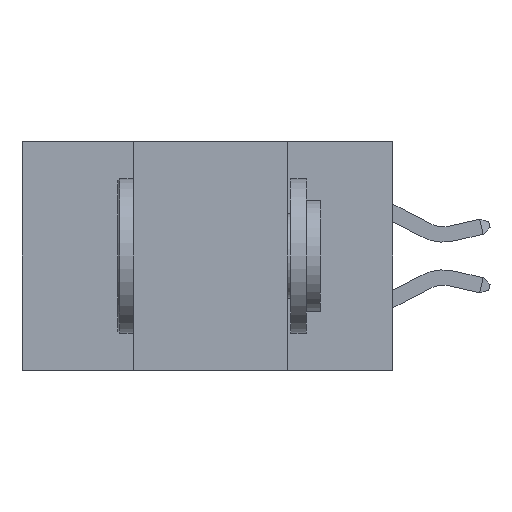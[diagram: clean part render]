
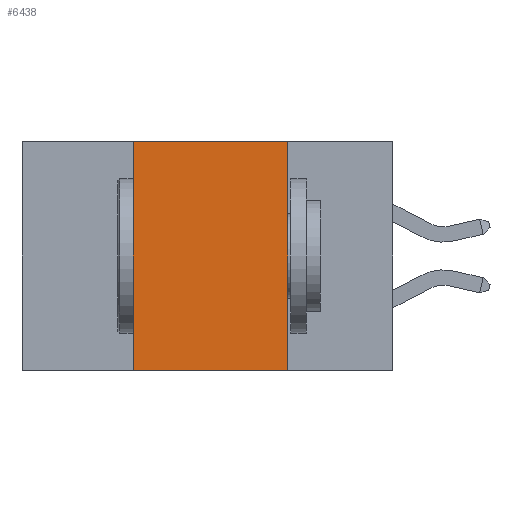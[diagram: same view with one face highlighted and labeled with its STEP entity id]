
A CAD part, left-side view. The second image highlights one B-rep face of the part: STEP entity #6438.
In plain terms, the highlighted planar face has unit normal (-1, 0, 0).
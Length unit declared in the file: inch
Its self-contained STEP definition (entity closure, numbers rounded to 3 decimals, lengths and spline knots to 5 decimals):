
#1858 = VERTEX_POINT ( 'NONE', #30913 ) ;
#2085 = DIRECTION ( 'NONE',  ( 0., 0., -1. ) ) ;
#2161 = VECTOR ( 'NONE', #22257, 39.37008 ) ;
#2575 = CARTESIAN_POINT ( 'NONE',  ( 0., 0.17, 0. ) ) ;
#4221 = DIRECTION ( 'NONE',  ( 0., 0., 1. ) ) ;
#5257 = DIRECTION ( 'NONE',  ( 0., 0., -1. ) ) ;
#6438 = ADVANCED_FACE ( 'NONE', ( #17389 ), #26666, .F. ) ;
#7757 = DIRECTION ( 'NONE',  ( 0., -1., 0. ) ) ;
#9501 = VECTOR ( 'NONE', #7757, 39.37008 ) ;
#10802 = VERTEX_POINT ( 'NONE', #17615 ) ;
#10861 = EDGE_CURVE ( 'NONE', #1858, #30908, #12055, .T. ) ;
#11122 = ORIENTED_EDGE ( 'NONE', *, *, #29031, .T. ) ;
#12055 = LINE ( 'NONE', #12930, #9501 ) ;
#12182 = VECTOR ( 'NONE', #5257, 39.37008 ) ;
#12930 = CARTESIAN_POINT ( 'NONE',  ( 0., 0.6, 0. ) ) ;
#13055 = LINE ( 'NONE', #30706, #2161 ) ;
#13828 = LINE ( 'NONE', #31190, #34319 ) ;
#15003 = ORIENTED_EDGE ( 'NONE', *, *, #29525, .F. ) ;
#17043 = ORIENTED_EDGE ( 'NONE', *, *, #19984, .F. ) ;
#17389 = FACE_OUTER_BOUND ( 'NONE', #31672, .T. ) ;
#17615 = CARTESIAN_POINT ( 'NONE',  ( 0., 0.42, -0.37 ) ) ;
#19984 = EDGE_CURVE ( 'NONE', #10802, #1858, #13828, .T. ) ;
#22257 = DIRECTION ( 'NONE',  ( 0., -1., 0. ) ) ;
#23313 = ORIENTED_EDGE ( 'NONE', *, *, #10861, .F. ) ;
#24729 = LINE ( 'NONE', #2575, #12182 ) ;
#26666 = PLANE ( 'NONE',  #34506 ) ;
#29031 = EDGE_CURVE ( 'NONE', #10802, #31333, #13055, .T. ) ;
#29327 = CARTESIAN_POINT ( 'NONE',  ( 0., 0.6, 0. ) ) ;
#29525 = EDGE_CURVE ( 'NONE', #30908, #31333, #24729, .T. ) ;
#30706 = CARTESIAN_POINT ( 'NONE',  ( 0., 0.6, -0.37 ) ) ;
#30908 = VERTEX_POINT ( 'NONE', #33503 ) ;
#30913 = CARTESIAN_POINT ( 'NONE',  ( 0., 0.42, 0. ) ) ;
#31190 = CARTESIAN_POINT ( 'NONE',  ( 0., 0.42, 0. ) ) ;
#31333 = VERTEX_POINT ( 'NONE', #34521 ) ;
#31672 = EDGE_LOOP ( 'NONE', ( #15003, #23313, #17043, #11122 ) ) ;
#33503 = CARTESIAN_POINT ( 'NONE',  ( 0., 0.17, 0. ) ) ;
#34244 = DIRECTION ( 'NONE',  ( 1., 0., 0. ) ) ;
#34319 = VECTOR ( 'NONE', #4221, 39.37008 ) ;
#34506 = AXIS2_PLACEMENT_3D ( 'NONE', #29327, #34244, #2085 ) ;
#34521 = CARTESIAN_POINT ( 'NONE',  ( 0., 0.17, -0.37 ) ) ;
